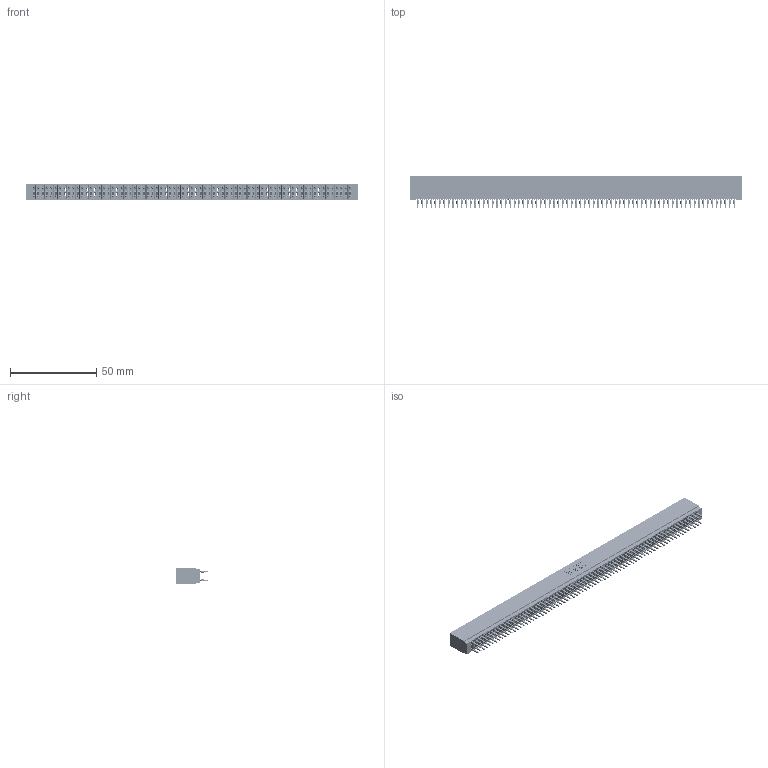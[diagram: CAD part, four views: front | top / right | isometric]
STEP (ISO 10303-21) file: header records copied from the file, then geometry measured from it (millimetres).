
FILE_DESCRIPTION (( 'STEP AP203' ), '1' );
FILE_NAME ('725-146-560-201.STEP', '2026-02-25T22:10:50', ( '' ), ( '' ), 'SwSTEP 2.0', 'SolidWorks 2023', '' );
FILE_SCHEMA (( 'CONFIG_CONTROL_DESIGN' ));
Length unit declared in the file: millimetre
Products named in the file (3): 745-292-001_560; 725 Part_Insulator Option - 01; 725-146-560-201
Assembly tree (147 placements, depth 2):
  725-146-560-201
    725 Part_Insulator Option - 01
    745-292-001_560  x146
Bounding box: 192.02 x 18.8 x 8.89 mm (x, y, z)
Volume: 15610.9 mm3; surface area: 35937.2 mm2
Topology: 147 solids, 147 shells, 14476 faces, 39601 edges, 25134 vertices
Faces by surface type: plane 7501, cylinder 3179, bspline 2920, torus 876
Entity records: 118952 total; most frequent: CARTESIAN_POINT 21125, ORIENTED_EDGE 20622, DIRECTION 17995, EDGE_CURVE 10311, VECTOR 9683, LINE 9683, VERTEX_POINT 6574, AXIS2_PLACEMENT_3D 4156
